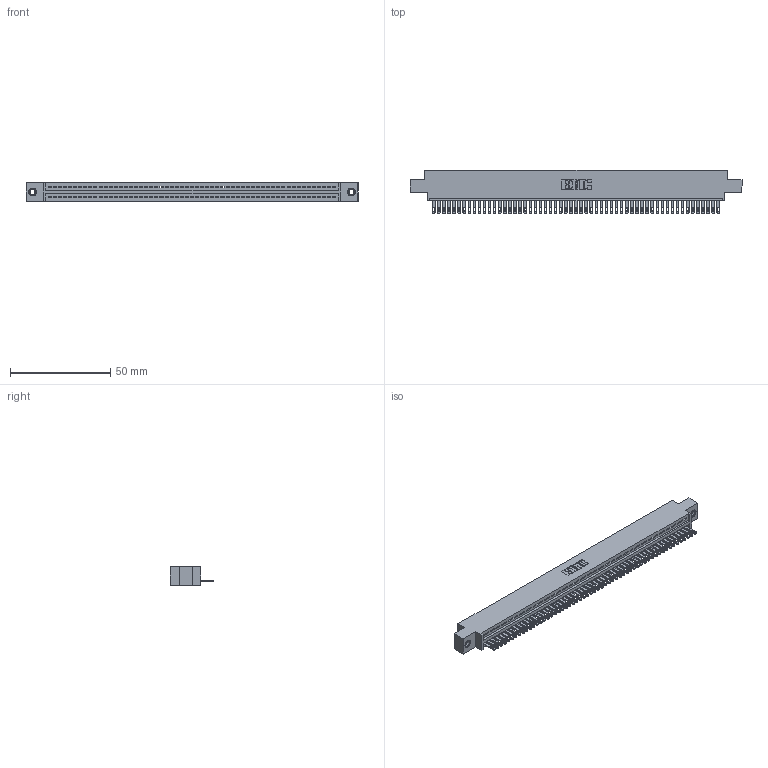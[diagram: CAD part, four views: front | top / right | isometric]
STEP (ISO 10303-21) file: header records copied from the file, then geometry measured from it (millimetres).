
FILE_DESCRIPTION (( 'STEP AP203' ), '1' );
FILE_NAME ('345-057-500-607.STEP', '2018-09-25T21:43:06', ( '' ), ( '' ), 'SwSTEP 2.0', 'SolidWorks 2016', '' );
FILE_SCHEMA (( 'CONFIG_CONTROL_DESIGN' ));
Length unit declared in the file: inch
Products named in the file (4): 345-250-001_345-250-005-103; 345-057-500-607; 345-292-001_345-293-100; 345 Part_0.170 Offset - 0.156 Dia-TI
Assembly tree (60 placements, depth 2):
  345-057-500-607
    345 Part_0.170 Offset - 0.156 Dia-TI
    345-292-001_345-293-100  x57
    345-250-001_345-250-005-103  x2
Bounding box: 165.99 x 21.51 x 9.4 mm (x, y, z)
Volume: 15797.1 mm3; surface area: 21483.8 mm2
Topology: 60 solids, 60 shells, 3268 faces, 10065 edges, 6702 vertices
Faces by surface type: plane 2054, cylinder 1198, cone 12, torus 4
Entity records: 42128 total; most frequent: CARTESIAN_POINT 7278, ORIENTED_EDGE 7262, DIRECTION 6363, EDGE_CURVE 3631, VECTOR 3247, LINE 3247, VERTEX_POINT 2416, AXIS2_PLACEMENT_3D 1558
